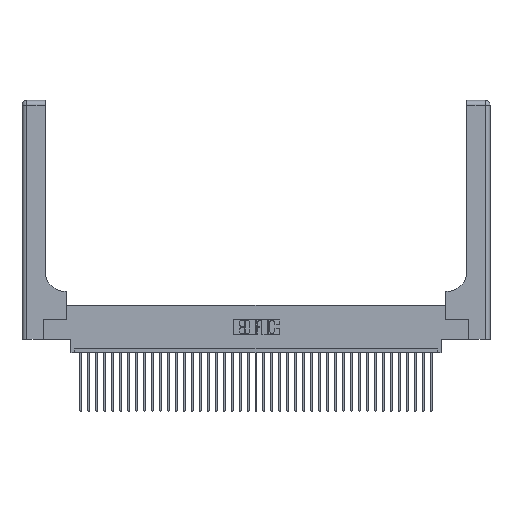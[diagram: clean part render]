
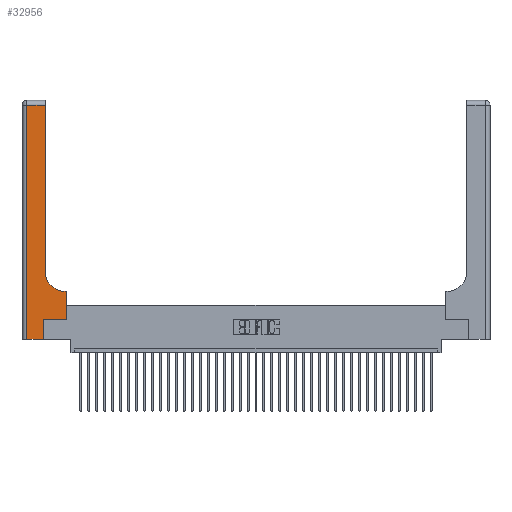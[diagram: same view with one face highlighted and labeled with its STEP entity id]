
A CAD part, top view. The second image highlights one B-rep face of the part: STEP entity #32956.
In plain terms, the highlighted planar face has unit normal (0, 0, 1).
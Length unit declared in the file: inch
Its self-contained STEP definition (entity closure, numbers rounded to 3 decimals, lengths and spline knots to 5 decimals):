
#8 = EDGE_LOOP ( 'NONE', ( #3798, #7076, #6621, #29475, #24690, #18330, #582, #2659, #31016 ) ) ;
#520 = LINE ( 'NONE', #31489, #36162 ) ;
#582 = ORIENTED_EDGE ( 'NONE', *, *, #7878, .T. ) ;
#1104 = VERTEX_POINT ( 'NONE', #18408 ) ;
#1564 = EDGE_CURVE ( 'NONE', #15005, #1104, #22473, .T. ) ;
#1630 = LINE ( 'NONE', #35384, #17594 ) ;
#2145 = VECTOR ( 'NONE', #15682, 39.37008 ) ;
#2201 = PLANE ( 'NONE',  #5798 ) ;
#2392 = CARTESIAN_POINT ( 'NONE',  ( 0.269, 0.25, 0.37 ) ) ;
#2659 = ORIENTED_EDGE ( 'NONE', *, *, #3955, .T. ) ;
#3746 = EDGE_CURVE ( 'NONE', #15215, #7407, #19014, .T. ) ;
#3798 = ORIENTED_EDGE ( 'NONE', *, *, #3746, .T. ) ;
#3865 = DIRECTION ( 'NONE',  ( 0., 1., 0. ) ) ;
#3955 = EDGE_CURVE ( 'NONE', #25055, #10398, #35865, .T. ) ;
#5040 = EDGE_CURVE ( 'NONE', #10601, #15005, #1630, .T. ) ;
#5282 = DIRECTION ( 'NONE',  ( 0., 1., 0. ) ) ;
#5505 = VECTOR ( 'NONE', #19387, 39.37008 ) ;
#5740 = CARTESIAN_POINT ( 'NONE',  ( 0.2915, 2.94, 0.37 ) ) ;
#5751 = CARTESIAN_POINT ( 'NONE',  ( 0.5585, 0.6, 0.37 ) ) ;
#5798 = AXIS2_PLACEMENT_3D ( 'NONE', #11119, #8367, #31962 ) ;
#6621 = ORIENTED_EDGE ( 'NONE', *, *, #23082, .T. ) ;
#6639 = CARTESIAN_POINT ( 'NONE',  ( 0.2915, 3., 0.37 ) ) ;
#7076 = ORIENTED_EDGE ( 'NONE', *, *, #14386, .T. ) ;
#7407 = VERTEX_POINT ( 'NONE', #5740 ) ;
#7878 = EDGE_CURVE ( 'NONE', #1104, #25055, #21913, .T. ) ;
#8367 = DIRECTION ( 'NONE',  ( 0., 0., -1. ) ) ;
#8499 = DIRECTION ( 'NONE',  ( -1., 0., 0. ) ) ;
#9355 = CARTESIAN_POINT ( 'NONE',  ( 0.5415, 0.85, 0.37 ) ) ;
#10398 = VERTEX_POINT ( 'NONE', #36545 ) ;
#10601 = VERTEX_POINT ( 'NONE', #20786 ) ;
#11025 = CARTESIAN_POINT ( 'NONE',  ( 0.269, 0.25, 0.37 ) ) ;
#11032 = CIRCLE ( 'NONE', #21108, 0.25 ) ;
#11119 = CARTESIAN_POINT ( 'NONE',  ( 0., 3., 0.37 ) ) ;
#12080 = CARTESIAN_POINT ( 'NONE',  ( 0.06, 2.94, 0.37 ) ) ;
#12834 = DIRECTION ( 'NONE',  ( 1., 0., 0. ) ) ;
#13439 = LINE ( 'NONE', #16773, #5505 ) ;
#13988 = VECTOR ( 'NONE', #3865, 39.37008 ) ;
#14386 = EDGE_CURVE ( 'NONE', #7407, #21550, #19999, .T. ) ;
#14523 = VECTOR ( 'NONE', #12834, 39.37008 ) ;
#15005 = VERTEX_POINT ( 'NONE', #2392 ) ;
#15215 = VERTEX_POINT ( 'NONE', #22513 ) ;
#15530 = DIRECTION ( 'NONE',  ( 1., 0., 0. ) ) ;
#15682 = DIRECTION ( 'NONE',  ( 0., 1., 0. ) ) ;
#16773 = CARTESIAN_POINT ( 'NONE',  ( 0., 0., 0.37 ) ) ;
#17594 = VECTOR ( 'NONE', #5282, 39.37008 ) ;
#18140 = VECTOR ( 'NONE', #8499, 39.37008 ) ;
#18330 = ORIENTED_EDGE ( 'NONE', *, *, #1564, .T. ) ;
#18408 = CARTESIAN_POINT ( 'NONE',  ( 0.5585, 0.25, 0.37 ) ) ;
#19014 = LINE ( 'NONE', #6639, #2145 ) ;
#19387 = DIRECTION ( 'NONE',  ( 1., 0., 0. ) ) ;
#19784 = CARTESIAN_POINT ( 'NONE',  ( 0.06, 0., 0.37 ) ) ;
#19999 = LINE ( 'NONE', #20404, #18140 ) ;
#20390 = EDGE_CURVE ( 'NONE', #28953, #10601, #13439, .T. ) ;
#20404 = CARTESIAN_POINT ( 'NONE',  ( 0., 2.94, 0.37 ) ) ;
#20786 = CARTESIAN_POINT ( 'NONE',  ( 0.269, 0., 0.37 ) ) ;
#21083 = FACE_OUTER_BOUND ( 'NONE', #8, .T. ) ;
#21108 = AXIS2_PLACEMENT_3D ( 'NONE', #9355, #21621, #15530 ) ;
#21550 = VERTEX_POINT ( 'NONE', #12080 ) ;
#21621 = DIRECTION ( 'NONE',  ( 0., 0., -1. ) ) ;
#21783 = CARTESIAN_POINT ( 'NONE',  ( 0.5585, 0.25, 0.37 ) ) ;
#21913 = LINE ( 'NONE', #21783, #13988 ) ;
#22473 = LINE ( 'NONE', #11025, #14523 ) ;
#22513 = CARTESIAN_POINT ( 'NONE',  ( 0.2915, 0.85, 0.37 ) ) ;
#22552 = DIRECTION ( 'NONE',  ( 0., -1., 0. ) ) ;
#23082 = EDGE_CURVE ( 'NONE', #21550, #28953, #520, .T. ) ;
#23144 = CARTESIAN_POINT ( 'NONE',  ( 0.2915, 0.6, 0.37 ) ) ;
#24690 = ORIENTED_EDGE ( 'NONE', *, *, #5040, .T. ) ;
#25055 = VERTEX_POINT ( 'NONE', #5751 ) ;
#28953 = VERTEX_POINT ( 'NONE', #19784 ) ;
#29475 = ORIENTED_EDGE ( 'NONE', *, *, #20390, .T. ) ;
#31016 = ORIENTED_EDGE ( 'NONE', *, *, #35725, .T. ) ;
#31489 = CARTESIAN_POINT ( 'NONE',  ( 0.06, 3., 0.37 ) ) ;
#31687 = VECTOR ( 'NONE', #34912, 39.37008 ) ;
#31962 = DIRECTION ( 'NONE',  ( -1., 0., 0. ) ) ;
#32956 = ADVANCED_FACE ( 'NONE', ( #21083 ), #2201, .F. ) ;
#34912 = DIRECTION ( 'NONE',  ( -1., 0., 0. ) ) ;
#35384 = CARTESIAN_POINT ( 'NONE',  ( 0.269, 0., 0.37 ) ) ;
#35725 = EDGE_CURVE ( 'NONE', #10398, #15215, #11032, .T. ) ;
#35865 = LINE ( 'NONE', #23144, #31687 ) ;
#36162 = VECTOR ( 'NONE', #22552, 39.37008 ) ;
#36545 = CARTESIAN_POINT ( 'NONE',  ( 0.5415, 0.6, 0.37 ) ) ;
